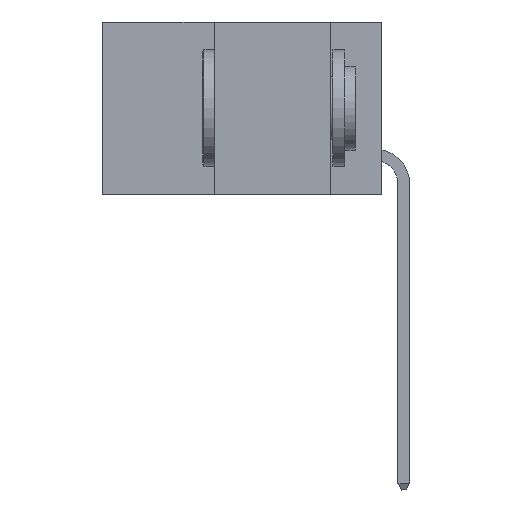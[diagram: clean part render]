
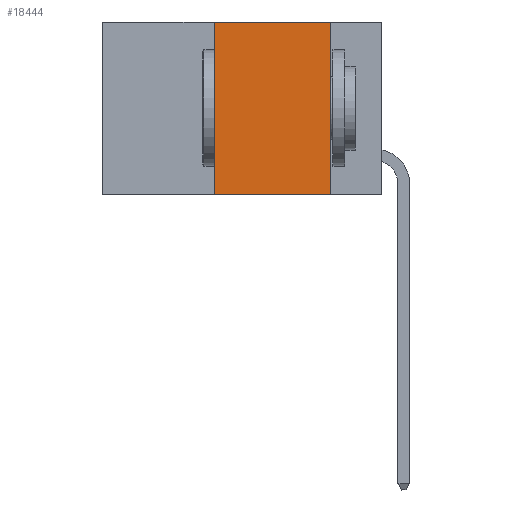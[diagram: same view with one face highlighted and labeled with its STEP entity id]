
A CAD part, left-side view. The second image highlights one B-rep face of the part: STEP entity #18444.
In plain terms, the highlighted planar face has unit normal (-1, 0, 0).
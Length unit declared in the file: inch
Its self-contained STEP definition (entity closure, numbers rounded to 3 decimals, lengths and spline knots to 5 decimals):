
#128 = EDGE_CURVE ( 'NONE', #4754, #7412, #11283, .T. ) ;
#1106 = DIRECTION ( 'NONE',  ( 0., 0., -1. ) ) ;
#1270 = DIRECTION ( 'NONE',  ( 0., 0., 1. ) ) ;
#1396 = ORIENTED_EDGE ( 'NONE', *, *, #5602, .F. ) ;
#2759 = ORIENTED_EDGE ( 'NONE', *, *, #15351, .F. ) ;
#2771 = EDGE_CURVE ( 'NONE', #4072, #7412, #14862, .T. ) ;
#3976 = CARTESIAN_POINT ( 'NONE',  ( 0., 0.6, 0. ) ) ;
#4072 = VERTEX_POINT ( 'NONE', #12825 ) ;
#4717 = LINE ( 'NONE', #8028, #16566 ) ;
#4754 = VERTEX_POINT ( 'NONE', #17728 ) ;
#4878 = DIRECTION ( 'NONE',  ( 0., 0., -1. ) ) ;
#5044 = CARTESIAN_POINT ( 'NONE',  ( 0., 0.6, -0.37 ) ) ;
#5094 = EDGE_LOOP ( 'NONE', ( #14937, #1396, #2759, #8127 ) ) ;
#5602 = EDGE_CURVE ( 'NONE', #14578, #4072, #4717, .T. ) ;
#5825 = CARTESIAN_POINT ( 'NONE',  ( 0., 0.11, -0.37 ) ) ;
#7412 = VERTEX_POINT ( 'NONE', #5825 ) ;
#7621 = VECTOR ( 'NONE', #16609, 39.37008 ) ;
#8028 = CARTESIAN_POINT ( 'NONE',  ( 0., 0.6, 0. ) ) ;
#8127 = ORIENTED_EDGE ( 'NONE', *, *, #128, .T. ) ;
#9488 = CARTESIAN_POINT ( 'NONE',  ( 0., 0.36, 0. ) ) ;
#10123 = AXIS2_PLACEMENT_3D ( 'NONE', #3976, #10882, #4878 ) ;
#10768 = PLANE ( 'NONE',  #10123 ) ;
#10882 = DIRECTION ( 'NONE',  ( 1., 0., 0. ) ) ;
#11283 = LINE ( 'NONE', #5044, #7621 ) ;
#12524 = CARTESIAN_POINT ( 'NONE',  ( 0., 0.11, 0. ) ) ;
#12825 = CARTESIAN_POINT ( 'NONE',  ( 0., 0.11, 0. ) ) ;
#13187 = LINE ( 'NONE', #18358, #16551 ) ;
#14578 = VERTEX_POINT ( 'NONE', #9488 ) ;
#14639 = VECTOR ( 'NONE', #1106, 39.37008 ) ;
#14862 = LINE ( 'NONE', #12524, #14639 ) ;
#14937 = ORIENTED_EDGE ( 'NONE', *, *, #2771, .F. ) ;
#15337 = DIRECTION ( 'NONE',  ( 0., -1., 0. ) ) ;
#15351 = EDGE_CURVE ( 'NONE', #4754, #14578, #13187, .T. ) ;
#16551 = VECTOR ( 'NONE', #1270, 39.37008 ) ;
#16566 = VECTOR ( 'NONE', #15337, 39.37008 ) ;
#16609 = DIRECTION ( 'NONE',  ( 0., -1., 0. ) ) ;
#17728 = CARTESIAN_POINT ( 'NONE',  ( 0., 0.36, -0.37 ) ) ;
#17839 = FACE_OUTER_BOUND ( 'NONE', #5094, .T. ) ;
#18358 = CARTESIAN_POINT ( 'NONE',  ( 0., 0.36, 0. ) ) ;
#18444 = ADVANCED_FACE ( 'NONE', ( #17839 ), #10768, .F. ) ;
